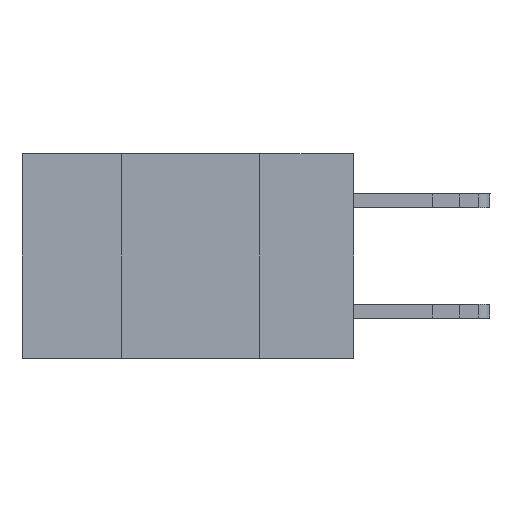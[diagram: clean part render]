
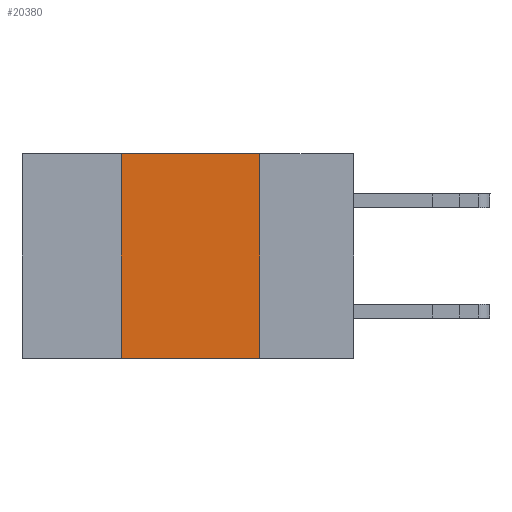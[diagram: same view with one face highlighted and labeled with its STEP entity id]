
A CAD part, left-side view. The second image highlights one B-rep face of the part: STEP entity #20380.
In plain terms, the highlighted planar face has unit normal (-1, 0, 0).
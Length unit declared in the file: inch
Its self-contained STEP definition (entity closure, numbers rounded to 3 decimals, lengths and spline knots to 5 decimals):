
#1207 = ORIENTED_EDGE ( 'NONE', *, *, #23418, .F. ) ;
#1525 = CARTESIAN_POINT ( 'NONE',  ( 0., 0.6, 0. ) ) ;
#3312 = CARTESIAN_POINT ( 'NONE',  ( 0., 0.42, 0. ) ) ;
#3642 = EDGE_CURVE ( 'NONE', #20826, #10174, #12775, .T. ) ;
#6200 = VECTOR ( 'NONE', #16690, 39.37008 ) ;
#6302 = CARTESIAN_POINT ( 'NONE',  ( 0., 0.6, 0. ) ) ;
#8491 = CARTESIAN_POINT ( 'NONE',  ( 0., 0.42, 0. ) ) ;
#9532 = FACE_OUTER_BOUND ( 'NONE', #10829, .T. ) ;
#10132 = DIRECTION ( 'NONE',  ( 1., 0., 0. ) ) ;
#10174 = VERTEX_POINT ( 'NONE', #23211 ) ;
#10266 = VERTEX_POINT ( 'NONE', #8491 ) ;
#10377 = VECTOR ( 'NONE', #20417, 39.37008 ) ;
#10829 = EDGE_LOOP ( 'NONE', ( #1207, #20405, #13166, #11285 ) ) ;
#10965 = LINE ( 'NONE', #11062, #10377 ) ;
#11062 = CARTESIAN_POINT ( 'NONE',  ( 0., 0.17, 0. ) ) ;
#11285 = ORIENTED_EDGE ( 'NONE', *, *, #3642, .T. ) ;
#11927 = CARTESIAN_POINT ( 'NONE',  ( 0., 0.17, 0. ) ) ;
#12775 = LINE ( 'NONE', #23952, #17149 ) ;
#12915 = AXIS2_PLACEMENT_3D ( 'NONE', #6302, #10132, #23289 ) ;
#13166 = ORIENTED_EDGE ( 'NONE', *, *, #16162, .F. ) ;
#14081 = LINE ( 'NONE', #3312, #19083 ) ;
#14538 = DIRECTION ( 'NONE',  ( 0., -1., 0. ) ) ;
#14602 = DIRECTION ( 'NONE',  ( 0., 0., 1. ) ) ;
#15007 = LINE ( 'NONE', #1525, #6200 ) ;
#15058 = EDGE_CURVE ( 'NONE', #10266, #15874, #15007, .T. ) ;
#15874 = VERTEX_POINT ( 'NONE', #11927 ) ;
#16162 = EDGE_CURVE ( 'NONE', #20826, #10266, #14081, .T. ) ;
#16690 = DIRECTION ( 'NONE',  ( 0., -1., 0. ) ) ;
#17149 = VECTOR ( 'NONE', #14538, 39.37008 ) ;
#17558 = PLANE ( 'NONE',  #12915 ) ;
#19083 = VECTOR ( 'NONE', #14602, 39.37008 ) ;
#20380 = ADVANCED_FACE ( 'NONE', ( #9532 ), #17558, .F. ) ;
#20405 = ORIENTED_EDGE ( 'NONE', *, *, #15058, .F. ) ;
#20417 = DIRECTION ( 'NONE',  ( 0., 0., -1. ) ) ;
#20826 = VERTEX_POINT ( 'NONE', #21210 ) ;
#21210 = CARTESIAN_POINT ( 'NONE',  ( 0., 0.42, -0.37 ) ) ;
#23211 = CARTESIAN_POINT ( 'NONE',  ( 0., 0.17, -0.37 ) ) ;
#23289 = DIRECTION ( 'NONE',  ( 0., 0., -1. ) ) ;
#23418 = EDGE_CURVE ( 'NONE', #15874, #10174, #10965, .T. ) ;
#23952 = CARTESIAN_POINT ( 'NONE',  ( 0., 0.6, -0.37 ) ) ;
